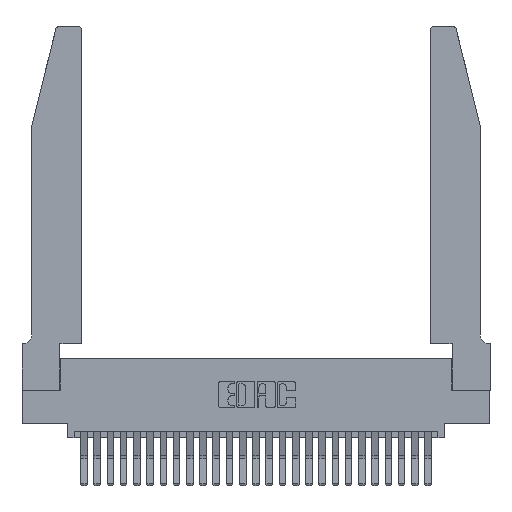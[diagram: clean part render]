
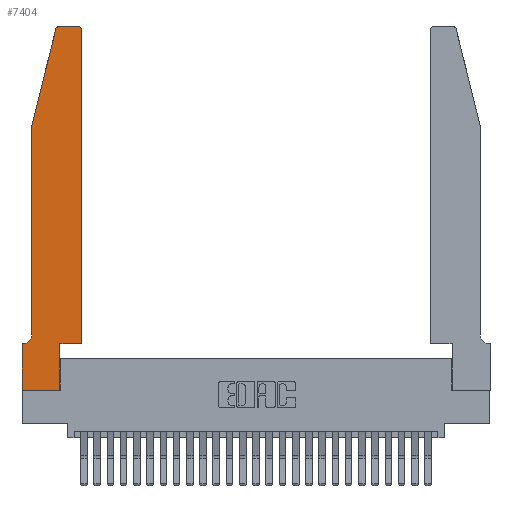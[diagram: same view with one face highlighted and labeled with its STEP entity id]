
A CAD part, top view. The second image highlights one B-rep face of the part: STEP entity #7404.
In plain terms, the highlighted planar face has unit normal (0, 0, 1).
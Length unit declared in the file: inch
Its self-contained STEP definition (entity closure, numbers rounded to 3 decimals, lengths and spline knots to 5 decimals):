
#25 = LINE ( 'NONE', #14032, #14240 ) ;
#157 = DIRECTION ( 'NONE',  ( -1., 0., 0. ) ) ;
#201 = EDGE_CURVE ( 'NONE', #13649, #18487, #26858, .T. ) ;
#278 = VERTEX_POINT ( 'NONE', #22040 ) ;
#676 = ORIENTED_EDGE ( 'NONE', *, *, #5454, .T. ) ;
#1195 = ORIENTED_EDGE ( 'NONE', *, *, #14713, .T. ) ;
#1654 = VERTEX_POINT ( 'NONE', #4330 ) ;
#1972 = ORIENTED_EDGE ( 'NONE', *, *, #25273, .T. ) ;
#2029 = VECTOR ( 'NONE', #3254, 39.37008 ) ;
#2207 = DIRECTION ( 'NONE',  ( 0., 0., 1. ) ) ;
#2539 = CARTESIAN_POINT ( 'NONE',  ( 0.0755, 2., 0.37 ) ) ;
#2687 = CARTESIAN_POINT ( 'NONE',  ( 0., 0.35, 0.37 ) ) ;
#2820 = CARTESIAN_POINT ( 'NONE',  ( 0.2605, 2.75, 0.37 ) ) ;
#2859 = CARTESIAN_POINT ( 'NONE',  ( 0.4205, 2.75, 0.37 ) ) ;
#3227 = DIRECTION ( 'NONE',  ( 0., 1., 0. ) ) ;
#3254 = DIRECTION ( 'NONE',  ( -0.239, -0.971, 0. ) ) ;
#3405 = CARTESIAN_POINT ( 'NONE',  ( 0.2865, 0.35, 0.37 ) ) ;
#4073 = CARTESIAN_POINT ( 'NONE',  ( 0.4505, 0.35, 0.37 ) ) ;
#4236 = VECTOR ( 'NONE', #11794, 39.37008 ) ;
#4330 = CARTESIAN_POINT ( 'NONE',  ( 0.25487, 2.72718, 0.37 ) ) ;
#4362 = DIRECTION ( 'NONE',  ( 1., 0., 0. ) ) ;
#4525 = ORIENTED_EDGE ( 'NONE', *, *, #17633, .T. ) ;
#4963 = CARTESIAN_POINT ( 'NONE',  ( 0.4205, 2.72, 0.37 ) ) ;
#5016 = EDGE_CURVE ( 'NONE', #7982, #15630, #25153, .T. ) ;
#5175 = ORIENTED_EDGE ( 'NONE', *, *, #25645, .T. ) ;
#5347 = CARTESIAN_POINT ( 'NONE',  ( 0., 0., 0.37 ) ) ;
#5454 = EDGE_CURVE ( 'NONE', #15630, #24867, #6389, .T. ) ;
#6142 = AXIS2_PLACEMENT_3D ( 'NONE', #15169, #2207, #4362 ) ;
#6370 = LINE ( 'NONE', #27378, #2029 ) ;
#6389 = LINE ( 'NONE', #13138, #22758 ) ;
#6894 = CIRCLE ( 'NONE', #16548, 0.03 ) ;
#6909 = LINE ( 'NONE', #5347, #4236 ) ;
#7404 = ADVANCED_FACE ( 'NONE', ( #22628 ), #27840, .T. ) ;
#7444 = LINE ( 'NONE', #4073, #14594 ) ;
#7764 = LINE ( 'NONE', #3405, #10501 ) ;
#7982 = VERTEX_POINT ( 'NONE', #24253 ) ;
#8073 = VECTOR ( 'NONE', #17599, 39.37008 ) ;
#8533 = DIRECTION ( 'NONE',  ( 0., 0., -1. ) ) ;
#8970 = EDGE_CURVE ( 'NONE', #15486, #20978, #6909, .T. ) ;
#9335 = CARTESIAN_POINT ( 'NONE',  ( 0.4505, 0.35, 0.37 ) ) ;
#10231 = EDGE_CURVE ( 'NONE', #19591, #7982, #20935, .T. ) ;
#10372 = CARTESIAN_POINT ( 'NONE',  ( 0.4505, 2.72, 0.37 ) ) ;
#10428 = DIRECTION ( 'NONE',  ( 0., 0., 1. ) ) ;
#10501 = VECTOR ( 'NONE', #3227, 39.37008 ) ;
#10631 = CIRCLE ( 'NONE', #6142, 0.03 ) ;
#11426 = EDGE_CURVE ( 'NONE', #1654, #19591, #6370, .T. ) ;
#11563 = AXIS2_PLACEMENT_3D ( 'NONE', #12836, #8533, #25887 ) ;
#11678 = VERTEX_POINT ( 'NONE', #14186 ) ;
#11794 = DIRECTION ( 'NONE',  ( 1., 0., 0. ) ) ;
#12270 = ORIENTED_EDGE ( 'NONE', *, *, #18659, .T. ) ;
#12654 = DIRECTION ( 'NONE',  ( 1., 0., 0. ) ) ;
#12831 = CARTESIAN_POINT ( 'NONE',  ( 0.0755, 2., 0.37 ) ) ;
#12836 = CARTESIAN_POINT ( 'NONE',  ( 0.0055, 0.42, 0.37 ) ) ;
#12995 = ORIENTED_EDGE ( 'NONE', *, *, #11426, .T. ) ;
#13138 = CARTESIAN_POINT ( 'NONE',  ( 0.0755, 0.35, 0.37 ) ) ;
#13649 = VERTEX_POINT ( 'NONE', #2859 ) ;
#14032 = CARTESIAN_POINT ( 'NONE',  ( 0., 0., 0.37 ) ) ;
#14186 = CARTESIAN_POINT ( 'NONE',  ( 0.4505, 0.35, 0.37 ) ) ;
#14240 = VECTOR ( 'NONE', #22328, 39.37008 ) ;
#14594 = VECTOR ( 'NONE', #17730, 39.37008 ) ;
#14713 = EDGE_CURVE ( 'NONE', #278, #11678, #16083, .T. ) ;
#15169 = CARTESIAN_POINT ( 'NONE',  ( 0.284, 2.72, 0.37 ) ) ;
#15486 = VERTEX_POINT ( 'NONE', #23341 ) ;
#15630 = VERTEX_POINT ( 'NONE', #23474 ) ;
#16083 = LINE ( 'NONE', #9335, #22580 ) ;
#16548 = AXIS2_PLACEMENT_3D ( 'NONE', #4963, #26580, #18201 ) ;
#16875 = CARTESIAN_POINT ( 'NONE',  ( 0.2865, 0., 0.37 ) ) ;
#16951 = CARTESIAN_POINT ( 'NONE',  ( 0., 0.35, 0.37 ) ) ;
#17599 = DIRECTION ( 'NONE',  ( -1., 0., 0. ) ) ;
#17633 = EDGE_CURVE ( 'NONE', #18487, #1654, #10631, .T. ) ;
#17730 = DIRECTION ( 'NONE',  ( 0., 1., 0. ) ) ;
#18006 = ORIENTED_EDGE ( 'NONE', *, *, #10231, .T. ) ;
#18201 = DIRECTION ( 'NONE',  ( 1., 0., 0. ) ) ;
#18487 = VERTEX_POINT ( 'NONE', #19812 ) ;
#18659 = EDGE_CURVE ( 'NONE', #27453, #13649, #6894, .T. ) ;
#19279 = ORIENTED_EDGE ( 'NONE', *, *, #8970, .T. ) ;
#19591 = VERTEX_POINT ( 'NONE', #2539 ) ;
#19812 = CARTESIAN_POINT ( 'NONE',  ( 0.284, 2.75, 0.37 ) ) ;
#20935 = LINE ( 'NONE', #12831, #21228 ) ;
#20978 = VERTEX_POINT ( 'NONE', #16875 ) ;
#21228 = VECTOR ( 'NONE', #23749, 39.37008 ) ;
#21997 = AXIS2_PLACEMENT_3D ( 'NONE', #16951, #10428, #12654 ) ;
#22040 = CARTESIAN_POINT ( 'NONE',  ( 0.2865, 0.35, 0.37 ) ) ;
#22138 = ORIENTED_EDGE ( 'NONE', *, *, #201, .T. ) ;
#22328 = DIRECTION ( 'NONE',  ( 0., -1., 0. ) ) ;
#22580 = VECTOR ( 'NONE', #27661, 39.37008 ) ;
#22628 = FACE_OUTER_BOUND ( 'NONE', #26273, .T. ) ;
#22758 = VECTOR ( 'NONE', #157, 39.37008 ) ;
#22928 = ORIENTED_EDGE ( 'NONE', *, *, #5016, .T. ) ;
#23341 = CARTESIAN_POINT ( 'NONE',  ( 0., 0., 0.37 ) ) ;
#23474 = CARTESIAN_POINT ( 'NONE',  ( 0.0055, 0.35, 0.37 ) ) ;
#23749 = DIRECTION ( 'NONE',  ( 0., -1., 0. ) ) ;
#24253 = CARTESIAN_POINT ( 'NONE',  ( 0.0755, 0.42, 0.37 ) ) ;
#24867 = VERTEX_POINT ( 'NONE', #2687 ) ;
#25153 = CIRCLE ( 'NONE', #11563, 0.07 ) ;
#25273 = EDGE_CURVE ( 'NONE', #11678, #27453, #7444, .T. ) ;
#25645 = EDGE_CURVE ( 'NONE', #20978, #278, #7764, .T. ) ;
#25887 = DIRECTION ( 'NONE',  ( -1., 0., 0. ) ) ;
#26101 = EDGE_CURVE ( 'NONE', #24867, #15486, #25, .T. ) ;
#26273 = EDGE_LOOP ( 'NONE', ( #22138, #4525, #12995, #18006, #22928, #676, #26353, #19279, #5175, #1195, #1972, #12270 ) ) ;
#26353 = ORIENTED_EDGE ( 'NONE', *, *, #26101, .T. ) ;
#26580 = DIRECTION ( 'NONE',  ( 0., 0., 1. ) ) ;
#26858 = LINE ( 'NONE', #2820, #8073 ) ;
#27378 = CARTESIAN_POINT ( 'NONE',  ( 0.0755, 2., 0.37 ) ) ;
#27453 = VERTEX_POINT ( 'NONE', #10372 ) ;
#27661 = DIRECTION ( 'NONE',  ( 1., 0., 0. ) ) ;
#27840 = PLANE ( 'NONE',  #21997 ) ;
